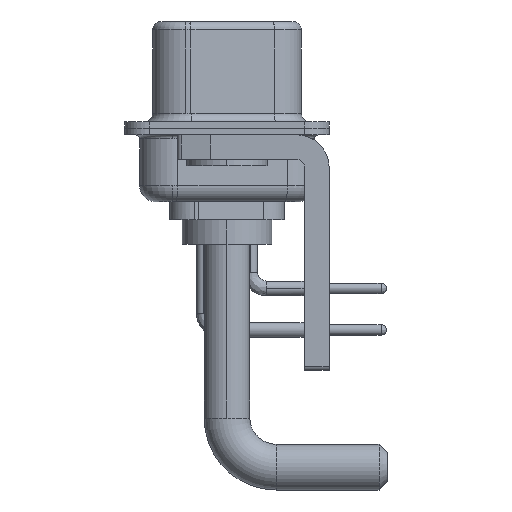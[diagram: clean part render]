
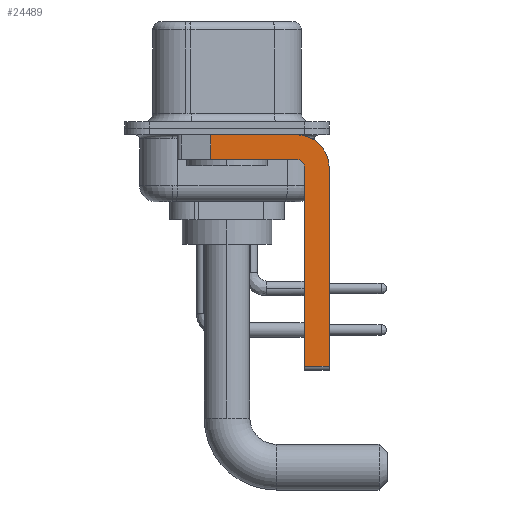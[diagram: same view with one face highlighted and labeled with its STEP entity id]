
A CAD part, left-side view. The second image highlights one B-rep face of the part: STEP entity #24489.
In plain terms, the highlighted planar face has unit normal (-1, 0, 0).
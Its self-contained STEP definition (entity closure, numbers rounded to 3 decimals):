
#186 = EDGE_CURVE ( 'NONE', #2114, #2097, #4137, .T. ) ;
#194 = DIRECTION ( 'NONE',  ( -1., 0., 0. ) ) ;
#540 = DIRECTION ( 'NONE',  ( 0., 1., 0. ) ) ;
#1315 = CARTESIAN_POINT ( 'NONE',  ( -2.9, -4.25, -2.4 ) ) ;
#1408 = PLANE ( 'NONE',  #12519 ) ;
#1413 = VECTOR ( 'NONE', #12401, 1000. ) ;
#1607 = VERTEX_POINT ( 'NONE', #19796 ) ;
#2097 = VERTEX_POINT ( 'NONE', #20000 ) ;
#2114 = VERTEX_POINT ( 'NONE', #17714 ) ;
#2565 = VECTOR ( 'NONE', #540, 1000. ) ;
#4137 = LINE ( 'NONE', #14007, #15110 ) ;
#4746 = EDGE_CURVE ( 'NONE', #1607, #21279, #15073, .T. ) ;
#4804 = ORIENTED_EDGE ( 'NONE', *, *, #25427, .F. ) ;
#4826 = CIRCLE ( 'NONE', #22719, 2. ) ;
#5105 = DIRECTION ( 'NONE',  ( 0., 0., 1. ) ) ;
#5506 = ORIENTED_EDGE ( 'NONE', *, *, #11248, .F. ) ;
#6512 = VERTEX_POINT ( 'NONE', #9173 ) ;
#7661 = VERTEX_POINT ( 'NONE', #14295 ) ;
#8326 = CARTESIAN_POINT ( 'NONE',  ( -2.9, 0.978, -1.9 ) ) ;
#8592 = DIRECTION ( 'NONE',  ( 0., 0., 1. ) ) ;
#9143 = EDGE_CURVE ( 'NONE', #2097, #14123, #4826, .T. ) ;
#9173 = CARTESIAN_POINT ( 'NONE',  ( -2.9, -6.25, -14.55 ) ) ;
#9541 = FACE_OUTER_BOUND ( 'NONE', #21647, .T. ) ;
#9579 = DIRECTION ( 'NONE',  ( 0., 0., -1. ) ) ;
#9680 = CARTESIAN_POINT ( 'NONE',  ( -2.9, -4.25, -2.4 ) ) ;
#10215 = LINE ( 'NONE', #20095, #10719 ) ;
#10404 = LINE ( 'NONE', #16267, #1413 ) ;
#10605 = DIRECTION ( 'NONE',  ( 0., 0., -1. ) ) ;
#10696 = ORIENTED_EDGE ( 'NONE', *, *, #9143, .F. ) ;
#10719 = VECTOR ( 'NONE', #13954, 1000. ) ;
#11248 = EDGE_CURVE ( 'NONE', #7661, #21103, #15257, .T. ) ;
#12401 = DIRECTION ( 'NONE',  ( 0., 0., -1. ) ) ;
#12519 = AXIS2_PLACEMENT_3D ( 'NONE', #9680, #17802, #25961 ) ;
#12866 = CARTESIAN_POINT ( 'NONE',  ( -2.9, 0.978, -1.9 ) ) ;
#13368 = ORIENTED_EDGE ( 'NONE', *, *, #22348, .T. ) ;
#13954 = DIRECTION ( 'NONE',  ( 0., -1., 0. ) ) ;
#14007 = CARTESIAN_POINT ( 'NONE',  ( -2.9, 3., -0.4 ) ) ;
#14123 = VERTEX_POINT ( 'NONE', #23176 ) ;
#14295 = CARTESIAN_POINT ( 'NONE',  ( -2.9, -4.75, -14.55 ) ) ;
#15073 = LINE ( 'NONE', #18816, #2565 ) ;
#15110 = VECTOR ( 'NONE', #20417, 1000. ) ;
#15257 = LINE ( 'NONE', #19002, #22434 ) ;
#15677 = LINE ( 'NONE', #8326, #20134 ) ;
#16204 = CARTESIAN_POINT ( 'NONE',  ( -2.9, -4.75, -2.4 ) ) ;
#16267 = CARTESIAN_POINT ( 'NONE',  ( -2.9, -6.25, -2.4 ) ) ;
#16707 = CIRCLE ( 'NONE', #20546, 0.5 ) ;
#17580 = DIRECTION ( 'NONE',  ( 1., 0., 0. ) ) ;
#17714 = CARTESIAN_POINT ( 'NONE',  ( -2.9, 0.978, -0.4 ) ) ;
#17801 = ORIENTED_EDGE ( 'NONE', *, *, #19824, .T. ) ;
#17802 = DIRECTION ( 'NONE',  ( 1., 0., 0. ) ) ;
#18295 = ORIENTED_EDGE ( 'NONE', *, *, #186, .F. ) ;
#18816 = CARTESIAN_POINT ( 'NONE',  ( -2.9, -4.25, -1.9 ) ) ;
#19002 = CARTESIAN_POINT ( 'NONE',  ( -2.9, -4.75, -14.8 ) ) ;
#19796 = CARTESIAN_POINT ( 'NONE',  ( -2.9, -4.25, -1.9 ) ) ;
#19824 = EDGE_CURVE ( 'NONE', #2114, #21279, #15677, .T. ) ;
#19841 = EDGE_CURVE ( 'NONE', #21103, #1607, #16707, .T. ) ;
#20000 = CARTESIAN_POINT ( 'NONE',  ( -2.9, -4.25, -0.4 ) ) ;
#20095 = CARTESIAN_POINT ( 'NONE',  ( -2.9, -4.25, -14.55 ) ) ;
#20134 = VECTOR ( 'NONE', #10605, 1000. ) ;
#20417 = DIRECTION ( 'NONE',  ( 0., -1., 0. ) ) ;
#20546 = AXIS2_PLACEMENT_3D ( 'NONE', #22350, #194, #8592 ) ;
#21103 = VERTEX_POINT ( 'NONE', #16204 ) ;
#21279 = VERTEX_POINT ( 'NONE', #12866 ) ;
#21647 = EDGE_LOOP ( 'NONE', ( #18295, #17801, #22247, #24170, #5506, #13368, #4804, #10696 ) ) ;
#22247 = ORIENTED_EDGE ( 'NONE', *, *, #4746, .F. ) ;
#22348 = EDGE_CURVE ( 'NONE', #7661, #6512, #10215, .T. ) ;
#22350 = CARTESIAN_POINT ( 'NONE',  ( -2.9, -4.25, -2.4 ) ) ;
#22434 = VECTOR ( 'NONE', #5105, 1000. ) ;
#22719 = AXIS2_PLACEMENT_3D ( 'NONE', #1315, #17580, #9579 ) ;
#23176 = CARTESIAN_POINT ( 'NONE',  ( -2.9, -6.25, -2.4 ) ) ;
#24170 = ORIENTED_EDGE ( 'NONE', *, *, #19841, .F. ) ;
#24489 = ADVANCED_FACE ( 'NONE', ( #9541 ), #1408, .F. ) ;
#25427 = EDGE_CURVE ( 'NONE', #14123, #6512, #10404, .T. ) ;
#25961 = DIRECTION ( 'NONE',  ( 0., 0., -1. ) ) ;
